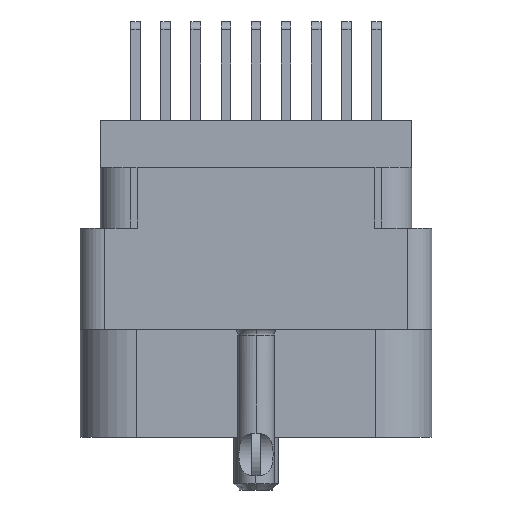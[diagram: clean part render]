
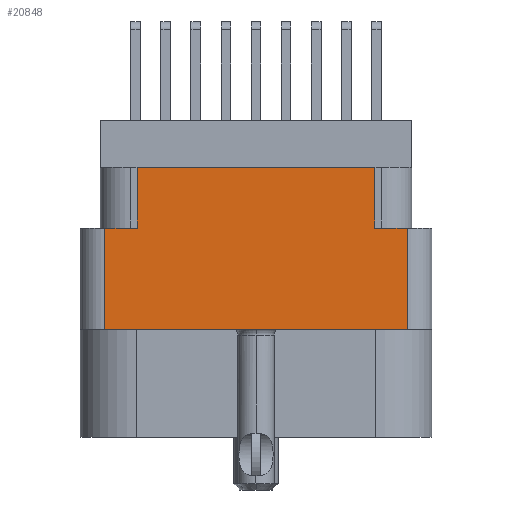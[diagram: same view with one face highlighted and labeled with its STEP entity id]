
A CAD part, left-side view. The second image highlights one B-rep face of the part: STEP entity #20848.
In plain terms, the highlighted planar face has unit normal (-1, 0, 0).
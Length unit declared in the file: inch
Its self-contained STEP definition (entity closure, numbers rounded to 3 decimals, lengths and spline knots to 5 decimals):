
#256 = VERTEX_POINT ( 'NONE', #26663 ) ;
#4906 = VECTOR ( 'NONE', #11445, 39.37008 ) ;
#4974 = EDGE_CURVE ( 'NONE', #44842, #39944, #22026, .T. ) ;
#6711 = LINE ( 'NONE', #24563, #8400 ) ;
#7733 = CARTESIAN_POINT ( 'NONE',  ( -1., 0.296, -0.117 ) ) ;
#7912 = DIRECTION ( 'NONE',  ( 0., -1., 0. ) ) ;
#7948 = VERTEX_POINT ( 'NONE', #31712 ) ;
#8029 = EDGE_CURVE ( 'NONE', #7948, #8946, #34097, .T. ) ;
#8400 = VECTOR ( 'NONE', #42656, 39.37008 ) ;
#8848 = DIRECTION ( 'NONE',  ( 0., 0., 1. ) ) ;
#8946 = VERTEX_POINT ( 'NONE', #40541 ) ;
#9417 = CARTESIAN_POINT ( 'NONE',  ( -1., -0.296, -0.117 ) ) ;
#10842 = VECTOR ( 'NONE', #44470, 39.37008 ) ;
#10945 = CARTESIAN_POINT ( 'NONE',  ( -1., -0.438, -0.789 ) ) ;
#11073 = VERTEX_POINT ( 'NONE', #20958 ) ;
#11445 = DIRECTION ( 'NONE',  ( 0., 0., -1. ) ) ;
#11945 = LINE ( 'NONE', #19331, #35210 ) ;
#12881 = CARTESIAN_POINT ( 'NONE',  ( -1., 0.296, -0.268 ) ) ;
#12944 = CARTESIAN_POINT ( 'NONE',  ( -1., -0.296, -0.268 ) ) ;
#15411 = ORIENTED_EDGE ( 'NONE', *, *, #16662, .T. ) ;
#16662 = EDGE_CURVE ( 'NONE', #35027, #7948, #36121, .T. ) ;
#16804 = EDGE_LOOP ( 'NONE', ( #44099, #15411, #22795, #24895, #18025, #18654, #31720, #41574 ) ) ;
#16914 = LINE ( 'NONE', #30431, #30486 ) ;
#17179 = AXIS2_PLACEMENT_3D ( 'NONE', #10945, #17969, #36171 ) ;
#17969 = DIRECTION ( 'NONE',  ( -1., 0., 0. ) ) ;
#18025 = ORIENTED_EDGE ( 'NONE', *, *, #21193, .F. ) ;
#18654 = ORIENTED_EDGE ( 'NONE', *, *, #32779, .T. ) ;
#19075 = VECTOR ( 'NONE', #37221, 39.37008 ) ;
#19331 = CARTESIAN_POINT ( 'NONE',  ( -1., 0., -0.268 ) ) ;
#20848 = ADVANCED_FACE ( 'NONE', ( #27131 ), #43655, .T. ) ;
#20958 = CARTESIAN_POINT ( 'NONE',  ( -1., -0.376, -0.268 ) ) ;
#21193 = EDGE_CURVE ( 'NONE', #256, #11073, #16914, .T. ) ;
#22026 = LINE ( 'NONE', #29901, #19075 ) ;
#22206 = VECTOR ( 'NONE', #31886, 39.37008 ) ;
#22795 = ORIENTED_EDGE ( 'NONE', *, *, #8029, .T. ) ;
#24563 = CARTESIAN_POINT ( 'NONE',  ( -1., -0.376, -0.789 ) ) ;
#24895 = ORIENTED_EDGE ( 'NONE', *, *, #40766, .T. ) ;
#25906 = CARTESIAN_POINT ( 'NONE',  ( -1., 0.376, -0.789 ) ) ;
#26663 = CARTESIAN_POINT ( 'NONE',  ( -1., -0.296, -0.268 ) ) ;
#27131 = FACE_OUTER_BOUND ( 'NONE', #16804, .T. ) ;
#29901 = CARTESIAN_POINT ( 'NONE',  ( -1., 0.296, -0.268 ) ) ;
#30051 = VERTEX_POINT ( 'NONE', #9417 ) ;
#30163 = CARTESIAN_POINT ( 'NONE',  ( -1., 0.438, -0.117 ) ) ;
#30431 = CARTESIAN_POINT ( 'NONE',  ( -1., 0., -0.268 ) ) ;
#30486 = VECTOR ( 'NONE', #37601, 39.37008 ) ;
#31712 = CARTESIAN_POINT ( 'NONE',  ( -1., 0.376, -0.52 ) ) ;
#31720 = ORIENTED_EDGE ( 'NONE', *, *, #38968, .F. ) ;
#31886 = DIRECTION ( 'NONE',  ( 0., -1., 0. ) ) ;
#32779 = EDGE_CURVE ( 'NONE', #256, #30051, #39362, .T. ) ;
#34097 = LINE ( 'NONE', #39499, #22206 ) ;
#35027 = VERTEX_POINT ( 'NONE', #38393 ) ;
#35210 = VECTOR ( 'NONE', #7912, 39.37008 ) ;
#36121 = LINE ( 'NONE', #25906, #4906 ) ;
#36171 = DIRECTION ( 'NONE',  ( 0., 0., 1. ) ) ;
#37221 = DIRECTION ( 'NONE',  ( 0., 0., 1. ) ) ;
#37601 = DIRECTION ( 'NONE',  ( 0., -1., 0. ) ) ;
#38393 = CARTESIAN_POINT ( 'NONE',  ( -1., 0.376, -0.268 ) ) ;
#38968 = EDGE_CURVE ( 'NONE', #39944, #30051, #42090, .T. ) ;
#39362 = LINE ( 'NONE', #12944, #45062 ) ;
#39499 = CARTESIAN_POINT ( 'NONE',  ( -1., 0., -0.52 ) ) ;
#39944 = VERTEX_POINT ( 'NONE', #7733 ) ;
#40541 = CARTESIAN_POINT ( 'NONE',  ( -1., -0.376, -0.52 ) ) ;
#40766 = EDGE_CURVE ( 'NONE', #8946, #11073, #6711, .T. ) ;
#41574 = ORIENTED_EDGE ( 'NONE', *, *, #4974, .F. ) ;
#42090 = LINE ( 'NONE', #30163, #10842 ) ;
#42656 = DIRECTION ( 'NONE',  ( 0., 0., 1. ) ) ;
#43655 = PLANE ( 'NONE',  #17179 ) ;
#44099 = ORIENTED_EDGE ( 'NONE', *, *, #44400, .F. ) ;
#44400 = EDGE_CURVE ( 'NONE', #35027, #44842, #11945, .T. ) ;
#44470 = DIRECTION ( 'NONE',  ( 0., -1., 0. ) ) ;
#44842 = VERTEX_POINT ( 'NONE', #12881 ) ;
#45062 = VECTOR ( 'NONE', #8848, 39.37008 ) ;
